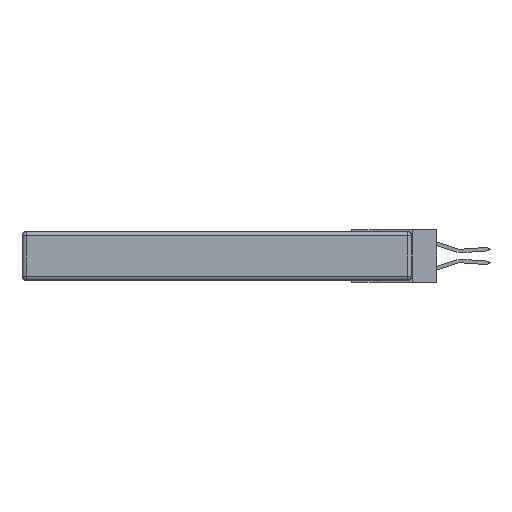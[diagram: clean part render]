
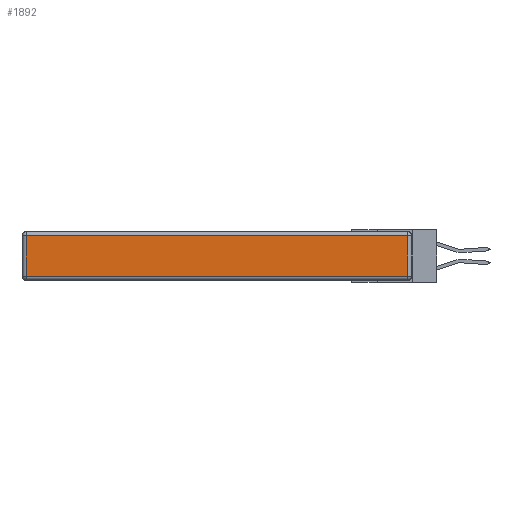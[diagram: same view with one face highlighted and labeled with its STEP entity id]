
A CAD part, left-side view. The second image highlights one B-rep face of the part: STEP entity #1892.
In plain terms, the highlighted planar face has unit normal (-1, 0, 0).
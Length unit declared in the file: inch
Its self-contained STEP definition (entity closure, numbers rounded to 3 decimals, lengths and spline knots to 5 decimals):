
#79 = VECTOR ( 'NONE', #16310, 39.37008 ) ;
#942 = EDGE_CURVE ( 'NONE', #8637, #3190, #21963, .T. ) ;
#1121 = ORIENTED_EDGE ( 'NONE', *, *, #15639, .T. ) ;
#1892 = ADVANCED_FACE ( 'NONE', ( #14043 ), #18002, .T. ) ;
#2036 = CARTESIAN_POINT ( 'NONE',  ( 0., 0.03, -0.03 ) ) ;
#2144 = AXIS2_PLACEMENT_3D ( 'NONE', #5274, #7040, #21898 ) ;
#2659 = CARTESIAN_POINT ( 'NONE',  ( 0., 2.75, -0.03 ) ) ;
#2750 = ORIENTED_EDGE ( 'NONE', *, *, #942, .T. ) ;
#3046 = EDGE_CURVE ( 'NONE', #12696, #8689, #4197, .T. ) ;
#3190 = VERTEX_POINT ( 'NONE', #7127 ) ;
#4197 = LINE ( 'NONE', #10207, #21818 ) ;
#4344 = EDGE_LOOP ( 'NONE', ( #1121, #19224, #20811, #2750 ) ) ;
#5274 = CARTESIAN_POINT ( 'NONE',  ( 0., 0., -0.343 ) ) ;
#7040 = DIRECTION ( 'NONE',  ( -1., 0., 0. ) ) ;
#7127 = CARTESIAN_POINT ( 'NONE',  ( 0., 2.72, -0.313 ) ) ;
#8637 = VERTEX_POINT ( 'NONE', #11156 ) ;
#8689 = VERTEX_POINT ( 'NONE', #2036 ) ;
#10207 = CARTESIAN_POINT ( 'NONE',  ( 0., 0.03, -0.343 ) ) ;
#10392 = DIRECTION ( 'NONE',  ( 0., 0., -1. ) ) ;
#11078 = CARTESIAN_POINT ( 'NONE',  ( 0., 0., -0.313 ) ) ;
#11156 = CARTESIAN_POINT ( 'NONE',  ( 0., 2.72, -0.03 ) ) ;
#12696 = VERTEX_POINT ( 'NONE', #21923 ) ;
#14043 = FACE_OUTER_BOUND ( 'NONE', #4344, .T. ) ;
#15639 = EDGE_CURVE ( 'NONE', #3190, #12696, #17645, .T. ) ;
#16310 = DIRECTION ( 'NONE',  ( 0., -1., 0. ) ) ;
#17008 = VECTOR ( 'NONE', #10392, 39.37008 ) ;
#17591 = EDGE_CURVE ( 'NONE', #8689, #8637, #22168, .T. ) ;
#17645 = LINE ( 'NONE', #11078, #79 ) ;
#18002 = PLANE ( 'NONE',  #2144 ) ;
#19224 = ORIENTED_EDGE ( 'NONE', *, *, #3046, .T. ) ;
#20811 = ORIENTED_EDGE ( 'NONE', *, *, #17591, .T. ) ;
#21818 = VECTOR ( 'NONE', #23127, 39.37008 ) ;
#21898 = DIRECTION ( 'NONE',  ( 0., 0., 1. ) ) ;
#21923 = CARTESIAN_POINT ( 'NONE',  ( 0., 0.03, -0.313 ) ) ;
#21963 = LINE ( 'NONE', #23576, #17008 ) ;
#22168 = LINE ( 'NONE', #2659, #22739 ) ;
#22739 = VECTOR ( 'NONE', #22849, 39.37008 ) ;
#22849 = DIRECTION ( 'NONE',  ( 0., 1., 0. ) ) ;
#23127 = DIRECTION ( 'NONE',  ( 0., 0., 1. ) ) ;
#23576 = CARTESIAN_POINT ( 'NONE',  ( 0., 2.72, -0.343 ) ) ;
